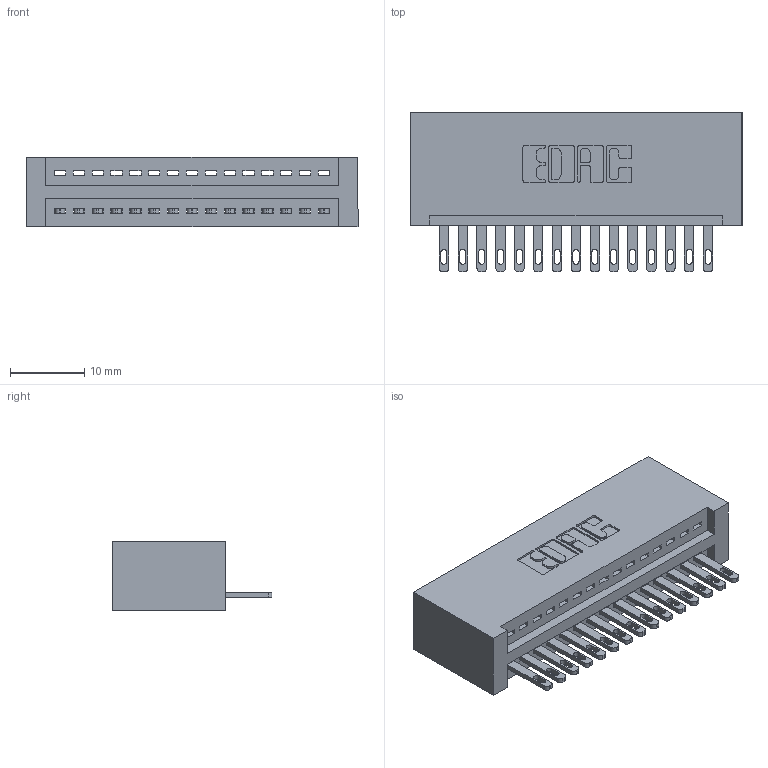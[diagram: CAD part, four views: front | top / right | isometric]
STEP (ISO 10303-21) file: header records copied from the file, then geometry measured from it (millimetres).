
FILE_DESCRIPTION (( 'STEP AP203' ), '1' );
FILE_NAME ('895-015-500-101.STEP', '2020-09-25T03:40:58', ( '' ), ( '' ), 'SwSTEP 2.0', 'SolidWorks 2020', '' );
FILE_SCHEMA (( 'CONFIG_CONTROL_DESIGN' ));
Length unit declared in the file: inch
Products named in the file (3): 845 Part_No Mounting Lugs; 895-015-500-101; 345-292-001_345-293-100
Assembly tree (16 placements, depth 2):
  895-015-500-101
    845 Part_No Mounting Lugs
    345-292-001_345-293-100  x15
Bounding box: 44.7 x 21.51 x 9.4 mm (x, y, z)
Volume: 4618.5 mm3; surface area: 5994.4 mm2
Topology: 16 solids, 16 shells, 928 faces, 2837 edges, 1890 vertices
Faces by surface type: plane 586, cylinder 342
Entity records: 14577 total; most frequent: CARTESIAN_POINT 2533, ORIENTED_EDGE 2482, DIRECTION 2247, EDGE_CURVE 1241, VECTOR 1053, LINE 1053, VERTEX_POINT 826, AXIS2_PLACEMENT_3D 597
